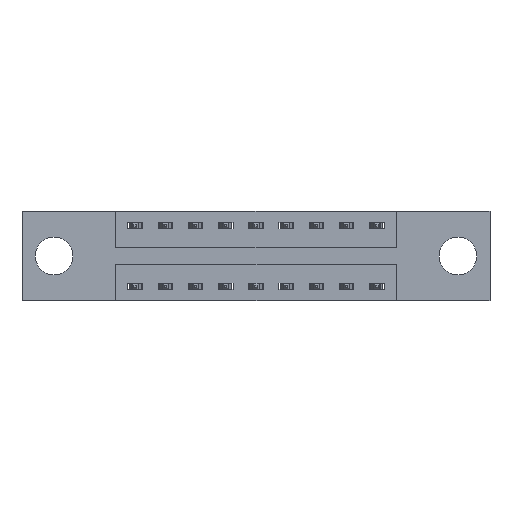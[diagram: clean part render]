
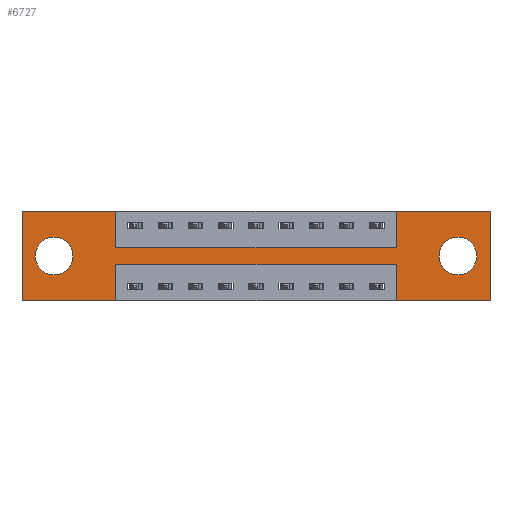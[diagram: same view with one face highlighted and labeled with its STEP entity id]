
A CAD part, front view. The second image highlights one B-rep face of the part: STEP entity #6727.
In plain terms, the highlighted planar face has unit normal (0, -1, 0).
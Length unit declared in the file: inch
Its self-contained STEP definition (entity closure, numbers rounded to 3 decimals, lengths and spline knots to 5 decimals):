
#4 = EDGE_CURVE ( 'NONE', #6443, #5323, #7594, .T. ) ;
#33 = VECTOR ( 'NONE', #6739, 39.37008 ) ;
#48 = EDGE_LOOP ( 'NONE', ( #3346, #7689, #9126, #7589, #2695, #958, #7680, #2602, #5560, #1043, #5904, #8105 ) ) ;
#152 = EDGE_CURVE ( 'NONE', #2835, #7094, #2531, .T. ) ;
#274 = VECTOR ( 'NONE', #772, 39.37008 ) ;
#385 = LINE ( 'NONE', #8641, #2114 ) ;
#391 = ORIENTED_EDGE ( 'NONE', *, *, #7512, .T. ) ;
#543 = CIRCLE ( 'NONE', #5354, 0.078 ) ;
#590 = CARTESIAN_POINT ( 'NONE',  ( 0., 0., -0.37 ) ) ;
#617 = CARTESIAN_POINT ( 'NONE',  ( 1.5475, 0., -0.37 ) ) ;
#660 = VERTEX_POINT ( 'NONE', #5905 ) ;
#747 = EDGE_LOOP ( 'NONE', ( #7556, #4254 ) ) ;
#772 = DIRECTION ( 'NONE',  ( 0., 0., 1. ) ) ;
#866 = DIRECTION ( 'NONE',  ( 0., 1., 0. ) ) ;
#957 = CARTESIAN_POINT ( 'NONE',  ( 0.1325, 0., -0.263 ) ) ;
#958 = ORIENTED_EDGE ( 'NONE', *, *, #5623, .F. ) ;
#1043 = ORIENTED_EDGE ( 'NONE', *, *, #2206, .F. ) ;
#1072 = DIRECTION ( 'NONE',  ( 0., 0., -1. ) ) ;
#1108 = EDGE_CURVE ( 'NONE', #5207, #6443, #9553, .T. ) ;
#1158 = VECTOR ( 'NONE', #8778, 39.37008 ) ;
#1717 = EDGE_CURVE ( 'NONE', #5323, #3796, #7942, .T. ) ;
#1824 = EDGE_CURVE ( 'NONE', #9182, #660, #2880, .T. ) ;
#1841 = EDGE_CURVE ( 'NONE', #7044, #5071, #9908, .T. ) ;
#1902 = CIRCLE ( 'NONE', #3388, 0.078 ) ;
#1917 = VECTOR ( 'NONE', #3175, 39.37008 ) ;
#2061 = CARTESIAN_POINT ( 'NONE',  ( 1.935, 0., 0. ) ) ;
#2114 = VECTOR ( 'NONE', #5148, 39.37008 ) ;
#2206 = EDGE_CURVE ( 'NONE', #3126, #2835, #385, .T. ) ;
#2377 = CARTESIAN_POINT ( 'NONE',  ( 1.935, 0., -0.37 ) ) ;
#2449 = EDGE_CURVE ( 'NONE', #5361, #3126, #5284, .T. ) ;
#2531 = LINE ( 'NONE', #6729, #4170 ) ;
#2602 = ORIENTED_EDGE ( 'NONE', *, *, #3799, .F. ) ;
#2637 = EDGE_CURVE ( 'NONE', #3796, #3562, #9785, .T. ) ;
#2638 = FACE_OUTER_BOUND ( 'NONE', #48, .T. ) ;
#2685 = VECTOR ( 'NONE', #4800, 39.37008 ) ;
#2695 = ORIENTED_EDGE ( 'NONE', *, *, #1108, .F. ) ;
#2835 = VERTEX_POINT ( 'NONE', #3186 ) ;
#2880 = CIRCLE ( 'NONE', #3439, 0.078 ) ;
#3060 = DIRECTION ( 'NONE',  ( -1., 0., 0. ) ) ;
#3126 = VERTEX_POINT ( 'NONE', #7522 ) ;
#3171 = VECTOR ( 'NONE', #8756, 39.37008 ) ;
#3175 = DIRECTION ( 'NONE',  ( -1., 0., 0. ) ) ;
#3186 = CARTESIAN_POINT ( 'NONE',  ( 0.3875, 0., 0. ) ) ;
#3237 = DIRECTION ( 'NONE',  ( 0., 0., 1. ) ) ;
#3262 = EDGE_LOOP ( 'NONE', ( #9828, #391 ) ) ;
#3346 = ORIENTED_EDGE ( 'NONE', *, *, #8897, .F. ) ;
#3388 = AXIS2_PLACEMENT_3D ( 'NONE', #10236, #7022, #7904 ) ;
#3439 = AXIS2_PLACEMENT_3D ( 'NONE', #5744, #866, #6435 ) ;
#3531 = VERTEX_POINT ( 'NONE', #9783 ) ;
#3562 = VERTEX_POINT ( 'NONE', #4291 ) ;
#3695 = CARTESIAN_POINT ( 'NONE',  ( 1.935, 0., 0. ) ) ;
#3708 = CARTESIAN_POINT ( 'NONE',  ( 0.3875, 0., -0.37 ) ) ;
#3796 = VERTEX_POINT ( 'NONE', #7002 ) ;
#3799 = EDGE_CURVE ( 'NONE', #7094, #4156, #9497, .T. ) ;
#3835 = CARTESIAN_POINT ( 'NONE',  ( 0., 0., -0.37 ) ) ;
#3988 = CARTESIAN_POINT ( 'NONE',  ( 0., 0., -0.37 ) ) ;
#4007 = CARTESIAN_POINT ( 'NONE',  ( 0.1325, 0., -0.185 ) ) ;
#4156 = VERTEX_POINT ( 'NONE', #6583 ) ;
#4170 = VECTOR ( 'NONE', #1072, 39.37008 ) ;
#4248 = CARTESIAN_POINT ( 'NONE',  ( 0.3875, 0., -0.22 ) ) ;
#4254 = ORIENTED_EDGE ( 'NONE', *, *, #1841, .T. ) ;
#4291 = CARTESIAN_POINT ( 'NONE',  ( 0.3875, 0., -0.22 ) ) ;
#4416 = FACE_BOUND ( 'NONE', #3262, .T. ) ;
#4537 = FACE_BOUND ( 'NONE', #747, .T. ) ;
#4627 = DIRECTION ( 'NONE',  ( 0., 0., -1. ) ) ;
#4690 = CARTESIAN_POINT ( 'NONE',  ( 0., 0., 0. ) ) ;
#4800 = DIRECTION ( 'NONE',  ( 1., 0., 0. ) ) ;
#4919 = CARTESIAN_POINT ( 'NONE',  ( 0.1325, 0., -0.107 ) ) ;
#5016 = LINE ( 'NONE', #7229, #7296 ) ;
#5071 = VERTEX_POINT ( 'NONE', #4919 ) ;
#5148 = DIRECTION ( 'NONE',  ( 1., 0., 0. ) ) ;
#5207 = VERTEX_POINT ( 'NONE', #3695 ) ;
#5284 = LINE ( 'NONE', #6281, #274 ) ;
#5323 = VERTEX_POINT ( 'NONE', #617 ) ;
#5354 = AXIS2_PLACEMENT_3D ( 'NONE', #5616, #8076, #5590 ) ;
#5361 = VERTEX_POINT ( 'NONE', #3988 ) ;
#5560 = ORIENTED_EDGE ( 'NONE', *, *, #152, .F. ) ;
#5590 = DIRECTION ( 'NONE',  ( 0., 0., -1. ) ) ;
#5616 = CARTESIAN_POINT ( 'NONE',  ( 1.8025, 0., -0.185 ) ) ;
#5623 = EDGE_CURVE ( 'NONE', #3531, #5207, #10083, .T. ) ;
#5644 = DIRECTION ( 'NONE',  ( 0., 1., 0. ) ) ;
#5744 = CARTESIAN_POINT ( 'NONE',  ( 1.8025, 0., -0.185 ) ) ;
#5833 = CARTESIAN_POINT ( 'NONE',  ( 0.3875, 0., -0.15 ) ) ;
#5904 = ORIENTED_EDGE ( 'NONE', *, *, #2449, .F. ) ;
#5905 = CARTESIAN_POINT ( 'NONE',  ( 1.8025, 0., -0.263 ) ) ;
#6164 = VERTEX_POINT ( 'NONE', #3708 ) ;
#6281 = CARTESIAN_POINT ( 'NONE',  ( 0., 0., 0. ) ) ;
#6435 = DIRECTION ( 'NONE',  ( 0., 0., -1. ) ) ;
#6443 = VERTEX_POINT ( 'NONE', #2377 ) ;
#6583 = CARTESIAN_POINT ( 'NONE',  ( 1.5475, 0., -0.15 ) ) ;
#6727 = ADVANCED_FACE ( 'NONE', ( #4416, #4537, #2638 ), #9443, .T. ) ;
#6729 = CARTESIAN_POINT ( 'NONE',  ( 0.3875, 0., 0. ) ) ;
#6739 = DIRECTION ( 'NONE',  ( 0., 0., -1. ) ) ;
#6861 = DIRECTION ( 'NONE',  ( 0., 0., -1. ) ) ;
#7002 = CARTESIAN_POINT ( 'NONE',  ( 1.5475, 0., -0.22 ) ) ;
#7022 = DIRECTION ( 'NONE',  ( 0., 1., 0. ) ) ;
#7044 = VERTEX_POINT ( 'NONE', #957 ) ;
#7094 = VERTEX_POINT ( 'NONE', #5833 ) ;
#7171 = VECTOR ( 'NONE', #3060, 39.37008 ) ;
#7229 = CARTESIAN_POINT ( 'NONE',  ( 1.5475, 0., 0. ) ) ;
#7296 = VECTOR ( 'NONE', #8747, 39.37008 ) ;
#7317 = CARTESIAN_POINT ( 'NONE',  ( 0., 0., -0.37 ) ) ;
#7364 = EDGE_CURVE ( 'NONE', #5071, #7044, #1902, .T. ) ;
#7512 = EDGE_CURVE ( 'NONE', #660, #9182, #543, .T. ) ;
#7522 = CARTESIAN_POINT ( 'NONE',  ( 0., 0., 0. ) ) ;
#7556 = ORIENTED_EDGE ( 'NONE', *, *, #7364, .T. ) ;
#7570 = VECTOR ( 'NONE', #6861, 39.37008 ) ;
#7589 = ORIENTED_EDGE ( 'NONE', *, *, #4, .F. ) ;
#7594 = LINE ( 'NONE', #7317, #1917 ) ;
#7669 = VECTOR ( 'NONE', #9356, 39.37008 ) ;
#7680 = ORIENTED_EDGE ( 'NONE', *, *, #10200, .F. ) ;
#7689 = ORIENTED_EDGE ( 'NONE', *, *, #2637, .F. ) ;
#7793 = LINE ( 'NONE', #3835, #7171 ) ;
#7904 = DIRECTION ( 'NONE',  ( 0., 0., 1. ) ) ;
#7942 = LINE ( 'NONE', #8018, #1158 ) ;
#8018 = CARTESIAN_POINT ( 'NONE',  ( 1.5475, 0., -0.37 ) ) ;
#8076 = DIRECTION ( 'NONE',  ( 0., 1., 0. ) ) ;
#8105 = ORIENTED_EDGE ( 'NONE', *, *, #8707, .F. ) ;
#8641 = CARTESIAN_POINT ( 'NONE',  ( 0., 0., 0. ) ) ;
#8707 = EDGE_CURVE ( 'NONE', #6164, #5361, #7793, .T. ) ;
#8747 = DIRECTION ( 'NONE',  ( 0., 0., 1. ) ) ;
#8756 = DIRECTION ( 'NONE',  ( 1., 0., 0. ) ) ;
#8778 = DIRECTION ( 'NONE',  ( 0., 0., 1. ) ) ;
#8881 = CARTESIAN_POINT ( 'NONE',  ( 1.8025, 0., -0.107 ) ) ;
#8897 = EDGE_CURVE ( 'NONE', #3562, #6164, #9534, .T. ) ;
#9126 = ORIENTED_EDGE ( 'NONE', *, *, #1717, .F. ) ;
#9129 = CARTESIAN_POINT ( 'NONE',  ( 0.3875, 0., -0.37 ) ) ;
#9182 = VERTEX_POINT ( 'NONE', #8881 ) ;
#9225 = CARTESIAN_POINT ( 'NONE',  ( 0.3875, 0., -0.15 ) ) ;
#9356 = DIRECTION ( 'NONE',  ( -1., 0., 0. ) ) ;
#9368 = AXIS2_PLACEMENT_3D ( 'NONE', #4007, #5644, #3237 ) ;
#9443 = PLANE ( 'NONE',  #10277 ) ;
#9497 = LINE ( 'NONE', #9225, #2685 ) ;
#9534 = LINE ( 'NONE', #9129, #33 ) ;
#9553 = LINE ( 'NONE', #2061, #7570 ) ;
#9783 = CARTESIAN_POINT ( 'NONE',  ( 1.5475, 0., 0. ) ) ;
#9785 = LINE ( 'NONE', #4248, #7669 ) ;
#9828 = ORIENTED_EDGE ( 'NONE', *, *, #1824, .T. ) ;
#9908 = CIRCLE ( 'NONE', #9368, 0.078 ) ;
#10083 = LINE ( 'NONE', #4690, #3171 ) ;
#10200 = EDGE_CURVE ( 'NONE', #4156, #3531, #5016, .T. ) ;
#10236 = CARTESIAN_POINT ( 'NONE',  ( 0.1325, 0., -0.185 ) ) ;
#10277 = AXIS2_PLACEMENT_3D ( 'NONE', #590, #10325, #4627 ) ;
#10325 = DIRECTION ( 'NONE',  ( 0., -1., 0. ) ) ;
